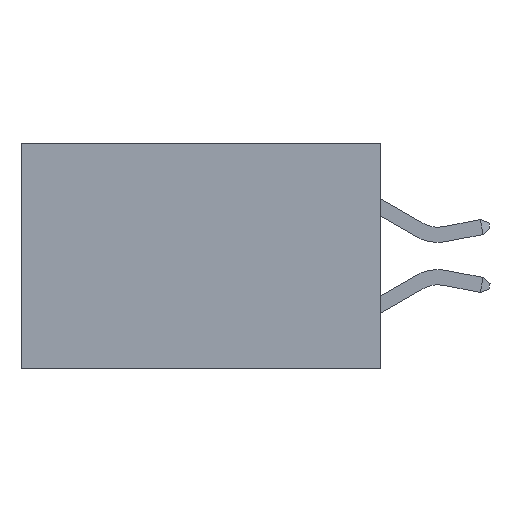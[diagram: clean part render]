
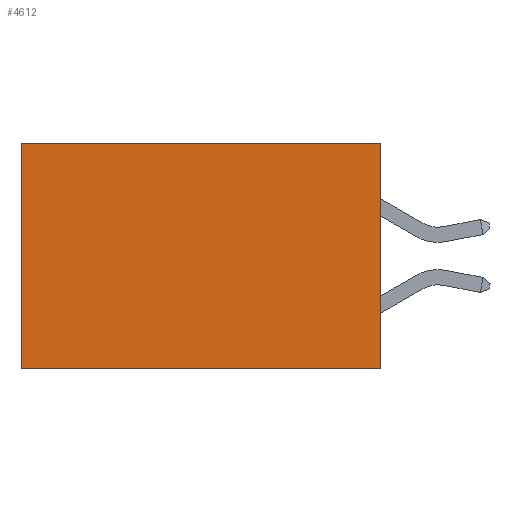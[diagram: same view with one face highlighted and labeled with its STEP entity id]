
A CAD part, left-side view. The second image highlights one B-rep face of the part: STEP entity #4612.
In plain terms, the highlighted planar face has unit normal (-1, 0, 0).
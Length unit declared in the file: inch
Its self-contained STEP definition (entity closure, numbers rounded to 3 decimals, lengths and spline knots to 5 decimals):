
#219 = LINE ( 'NONE', #6198, #9453 ) ;
#768 = LINE ( 'NONE', #8038, #10011 ) ;
#824 = VERTEX_POINT ( 'NONE', #3301 ) ;
#2075 = DIRECTION ( 'NONE',  ( 0., 1., 0. ) ) ;
#3301 = CARTESIAN_POINT ( 'NONE',  ( 0.277, 0., 0. ) ) ;
#3627 = ORIENTED_EDGE ( 'NONE', *, *, #8275, .T. ) ;
#3778 = VECTOR ( 'NONE', #3966, 39.37008 ) ;
#3903 = VECTOR ( 'NONE', #9888, 39.37008 ) ;
#3966 = DIRECTION ( 'NONE',  ( 0., 0., -1. ) ) ;
#4153 = LINE ( 'NONE', #13596, #3778 ) ;
#4612 = ADVANCED_FACE ( 'NONE', ( #4755 ), #13983, .F. ) ;
#4639 = ORIENTED_EDGE ( 'NONE', *, *, #6949, .F. ) ;
#4691 = DIRECTION ( 'NONE',  ( 0., 0., -1. ) ) ;
#4755 = FACE_OUTER_BOUND ( 'NONE', #14996, .T. ) ;
#6064 = EDGE_CURVE ( 'NONE', #14783, #9056, #219, .T. ) ;
#6198 = CARTESIAN_POINT ( 'NONE',  ( 0.277, 0.59, -0.37 ) ) ;
#6949 = EDGE_CURVE ( 'NONE', #824, #15271, #4153, .T. ) ;
#7464 = LINE ( 'NONE', #11105, #3903 ) ;
#8038 = CARTESIAN_POINT ( 'NONE',  ( 0.277, 0., -0.37 ) ) ;
#8275 = EDGE_CURVE ( 'NONE', #824, #14783, #7464, .T. ) ;
#8630 = ORIENTED_EDGE ( 'NONE', *, *, #6064, .T. ) ;
#9056 = VERTEX_POINT ( 'NONE', #14785 ) ;
#9453 = VECTOR ( 'NONE', #4691, 39.37008 ) ;
#9517 = AXIS2_PLACEMENT_3D ( 'NONE', #13885, #13805, #13771 ) ;
#9888 = DIRECTION ( 'NONE',  ( 0., 1., 0. ) ) ;
#10011 = VECTOR ( 'NONE', #2075, 39.37008 ) ;
#11105 = CARTESIAN_POINT ( 'NONE',  ( 0.277, 0., 0. ) ) ;
#11690 = CARTESIAN_POINT ( 'NONE',  ( 0.277, 0., -0.37 ) ) ;
#12027 = CARTESIAN_POINT ( 'NONE',  ( 0.277, 0.59, 0. ) ) ;
#12179 = EDGE_CURVE ( 'NONE', #15271, #9056, #768, .T. ) ;
#13596 = CARTESIAN_POINT ( 'NONE',  ( 0.277, 0., -0.37 ) ) ;
#13771 = DIRECTION ( 'NONE',  ( 0., 0., -1. ) ) ;
#13805 = DIRECTION ( 'NONE',  ( 1., 0., 0. ) ) ;
#13885 = CARTESIAN_POINT ( 'NONE',  ( 0.277, 0., -0.37 ) ) ;
#13983 = PLANE ( 'NONE',  #9517 ) ;
#14783 = VERTEX_POINT ( 'NONE', #12027 ) ;
#14785 = CARTESIAN_POINT ( 'NONE',  ( 0.277, 0.59, -0.37 ) ) ;
#14996 = EDGE_LOOP ( 'NONE', ( #8630, #15184, #4639, #3627 ) ) ;
#15184 = ORIENTED_EDGE ( 'NONE', *, *, #12179, .F. ) ;
#15271 = VERTEX_POINT ( 'NONE', #11690 ) ;
